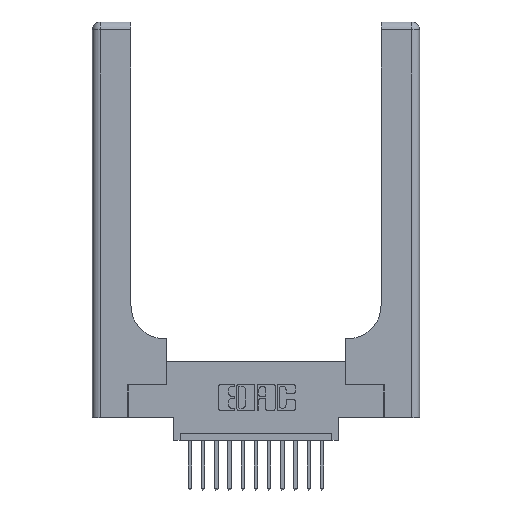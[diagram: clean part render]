
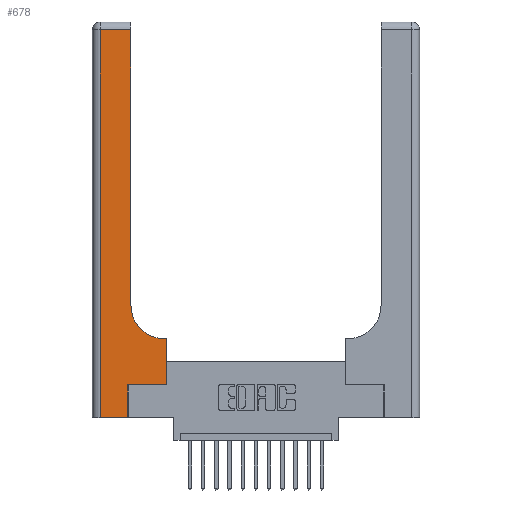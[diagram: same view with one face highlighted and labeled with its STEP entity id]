
A CAD part, top view. The second image highlights one B-rep face of the part: STEP entity #678.
In plain terms, the highlighted planar face has unit normal (0, 0, 1).
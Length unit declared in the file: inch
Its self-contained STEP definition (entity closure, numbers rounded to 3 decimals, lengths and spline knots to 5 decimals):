
#7 = PLANE ( 'NONE',  #1491 ) ;
#84 = VERTEX_POINT ( 'NONE', #6813 ) ;
#157 = VERTEX_POINT ( 'NONE', #8815 ) ;
#182 = CARTESIAN_POINT ( 'NONE',  ( 0.5415, 0.85, 0.37 ) ) ;
#237 = ORIENTED_EDGE ( 'NONE', *, *, #16750, .T. ) ;
#333 = CARTESIAN_POINT ( 'NONE',  ( 0.5585, 0.25, 0.37 ) ) ;
#423 = LINE ( 'NONE', #15702, #1932 ) ;
#546 = LINE ( 'NONE', #3798, #11501 ) ;
#610 = EDGE_CURVE ( 'NONE', #4557, #10817, #16243, .T. ) ;
#678 = ADVANCED_FACE ( 'NONE', ( #16450 ), #7, .F. ) ;
#1136 = VECTOR ( 'NONE', #3380, 39.37008 ) ;
#1356 = VERTEX_POINT ( 'NONE', #2585 ) ;
#1398 = DIRECTION ( 'NONE',  ( -1., 0., 0. ) ) ;
#1491 = AXIS2_PLACEMENT_3D ( 'NONE', #9571, #5616, #1398 ) ;
#1564 = EDGE_CURVE ( 'NONE', #7334, #4557, #2273, .T. ) ;
#1766 = VERTEX_POINT ( 'NONE', #12430 ) ;
#1932 = VECTOR ( 'NONE', #7594, 39.37008 ) ;
#2000 = CARTESIAN_POINT ( 'NONE',  ( 0.269, 0.25, 0.37 ) ) ;
#2273 = LINE ( 'NONE', #6900, #17059 ) ;
#2386 = ORIENTED_EDGE ( 'NONE', *, *, #14029, .T. ) ;
#2484 = ORIENTED_EDGE ( 'NONE', *, *, #1564, .T. ) ;
#2585 = CARTESIAN_POINT ( 'NONE',  ( 0.2915, 0.85, 0.37 ) ) ;
#3023 = CARTESIAN_POINT ( 'NONE',  ( 0.06, 3., 0.37 ) ) ;
#3290 = AXIS2_PLACEMENT_3D ( 'NONE', #182, #11113, #9807 ) ;
#3380 = DIRECTION ( 'NONE',  ( 1., 0., 0. ) ) ;
#3646 = LINE ( 'NONE', #14092, #17362 ) ;
#3798 = CARTESIAN_POINT ( 'NONE',  ( 0.2915, 0.6, 0.37 ) ) ;
#4557 = VERTEX_POINT ( 'NONE', #10103 ) ;
#5186 = DIRECTION ( 'NONE',  ( 1., 0., 0. ) ) ;
#5616 = DIRECTION ( 'NONE',  ( 0., 0., -1. ) ) ;
#5923 = DIRECTION ( 'NONE',  ( 0., -1., 0. ) ) ;
#6411 = VECTOR ( 'NONE', #5923, 39.37008 ) ;
#6741 = CARTESIAN_POINT ( 'NONE',  ( 0., 0., 0.37 ) ) ;
#6813 = CARTESIAN_POINT ( 'NONE',  ( 0.5585, 0.25, 0.37 ) ) ;
#6900 = CARTESIAN_POINT ( 'NONE',  ( 0., 2.94, 0.37 ) ) ;
#7334 = VERTEX_POINT ( 'NONE', #9270 ) ;
#7586 = ORIENTED_EDGE ( 'NONE', *, *, #15980, .T. ) ;
#7594 = DIRECTION ( 'NONE',  ( 0., 1., 0. ) ) ;
#8468 = LINE ( 'NONE', #2000, #1136 ) ;
#8673 = DIRECTION ( 'NONE',  ( 0., 1., 0. ) ) ;
#8815 = CARTESIAN_POINT ( 'NONE',  ( 0.269, 0.25, 0.37 ) ) ;
#9270 = CARTESIAN_POINT ( 'NONE',  ( 0.2915, 2.94, 0.37 ) ) ;
#9571 = CARTESIAN_POINT ( 'NONE',  ( 0., 3., 0.37 ) ) ;
#9807 = DIRECTION ( 'NONE',  ( 1., 0., 0. ) ) ;
#10090 = ORIENTED_EDGE ( 'NONE', *, *, #11717, .T. ) ;
#10103 = CARTESIAN_POINT ( 'NONE',  ( 0.06, 2.94, 0.37 ) ) ;
#10441 = ORIENTED_EDGE ( 'NONE', *, *, #10875, .T. ) ;
#10549 = ORIENTED_EDGE ( 'NONE', *, *, #10555, .T. ) ;
#10555 = EDGE_CURVE ( 'NONE', #16454, #1356, #13308, .T. ) ;
#10817 = VERTEX_POINT ( 'NONE', #14382 ) ;
#10875 = EDGE_CURVE ( 'NONE', #1766, #157, #423, .T. ) ;
#10903 = ORIENTED_EDGE ( 'NONE', *, *, #610, .T. ) ;
#11113 = DIRECTION ( 'NONE',  ( 0., 0., -1. ) ) ;
#11501 = VECTOR ( 'NONE', #11819, 39.37008 ) ;
#11717 = EDGE_CURVE ( 'NONE', #84, #15066, #11818, .T. ) ;
#11818 = LINE ( 'NONE', #333, #17395 ) ;
#11819 = DIRECTION ( 'NONE',  ( -1., 0., 0. ) ) ;
#12254 = EDGE_LOOP ( 'NONE', ( #15114, #2484, #10903, #237, #10441, #7586, #10090, #2386, #10549 ) ) ;
#12430 = CARTESIAN_POINT ( 'NONE',  ( 0.269, 0., 0.37 ) ) ;
#12667 = CARTESIAN_POINT ( 'NONE',  ( 0.5585, 0.6, 0.37 ) ) ;
#12815 = LINE ( 'NONE', #6741, #13652 ) ;
#13308 = CIRCLE ( 'NONE', #3290, 0.25 ) ;
#13652 = VECTOR ( 'NONE', #5186, 39.37008 ) ;
#13695 = DIRECTION ( 'NONE',  ( -1., 0., 0. ) ) ;
#14029 = EDGE_CURVE ( 'NONE', #15066, #16454, #546, .T. ) ;
#14092 = CARTESIAN_POINT ( 'NONE',  ( 0.2915, 3., 0.37 ) ) ;
#14382 = CARTESIAN_POINT ( 'NONE',  ( 0.06, 0., 0.37 ) ) ;
#15066 = VERTEX_POINT ( 'NONE', #12667 ) ;
#15114 = ORIENTED_EDGE ( 'NONE', *, *, #15915, .T. ) ;
#15702 = CARTESIAN_POINT ( 'NONE',  ( 0.269, 0., 0.37 ) ) ;
#15915 = EDGE_CURVE ( 'NONE', #1356, #7334, #3646, .T. ) ;
#15980 = EDGE_CURVE ( 'NONE', #157, #84, #8468, .T. ) ;
#16243 = LINE ( 'NONE', #3023, #6411 ) ;
#16450 = FACE_OUTER_BOUND ( 'NONE', #12254, .T. ) ;
#16454 = VERTEX_POINT ( 'NONE', #17691 ) ;
#16728 = DIRECTION ( 'NONE',  ( 0., 1., 0. ) ) ;
#16750 = EDGE_CURVE ( 'NONE', #10817, #1766, #12815, .T. ) ;
#17059 = VECTOR ( 'NONE', #13695, 39.37008 ) ;
#17362 = VECTOR ( 'NONE', #8673, 39.37008 ) ;
#17395 = VECTOR ( 'NONE', #16728, 39.37008 ) ;
#17691 = CARTESIAN_POINT ( 'NONE',  ( 0.5415, 0.6, 0.37 ) ) ;
